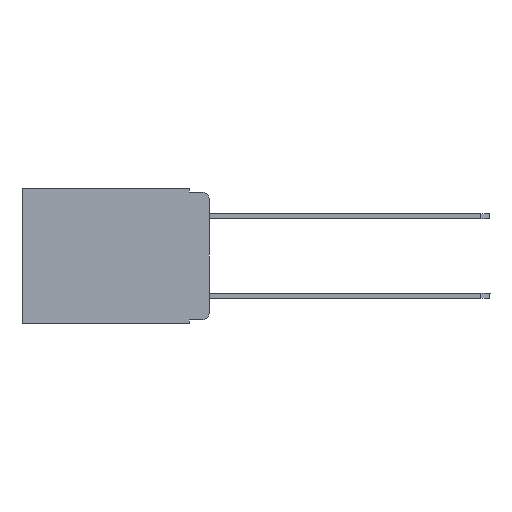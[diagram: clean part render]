
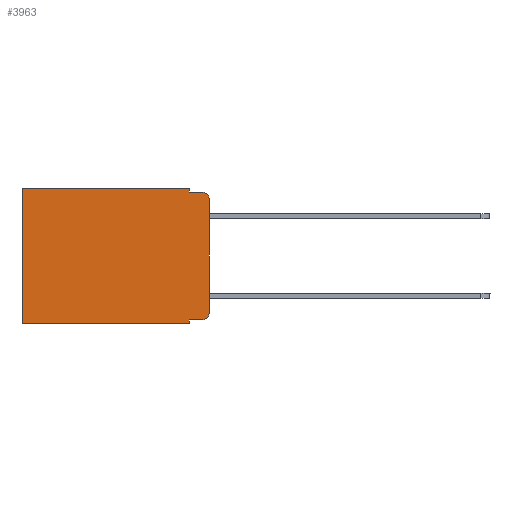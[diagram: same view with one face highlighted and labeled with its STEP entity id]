
A CAD part, left-side view. The second image highlights one B-rep face of the part: STEP entity #3963.
In plain terms, the highlighted planar face has unit normal (-1, 0, 0).
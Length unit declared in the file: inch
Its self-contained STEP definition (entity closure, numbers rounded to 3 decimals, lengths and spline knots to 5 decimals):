
#516 = DIRECTION ( 'NONE',  ( 0., -1., 0. ) ) ;
#684 = EDGE_CURVE ( 'NONE', #8232, #2446, #5012, .T. ) ;
#931 = DIRECTION ( 'NONE',  ( 0., 0., -1. ) ) ;
#959 = FACE_OUTER_BOUND ( 'NONE', #6966, .T. ) ;
#1146 = VERTEX_POINT ( 'NONE', #11413 ) ;
#1171 = AXIS2_PLACEMENT_3D ( 'NONE', #11766, #9076, #5073 ) ;
#1216 = ORIENTED_EDGE ( 'NONE', *, *, #16501, .T. ) ;
#1362 = EDGE_CURVE ( 'NONE', #7053, #8490, #6980, .T. ) ;
#1566 = ORIENTED_EDGE ( 'NONE', *, *, #14973, .T. ) ;
#1646 = VERTEX_POINT ( 'NONE', #10057 ) ;
#2324 = CARTESIAN_POINT ( 'NONE',  ( 0.298, 0.051, -0.01 ) ) ;
#2446 = VERTEX_POINT ( 'NONE', #9482 ) ;
#2644 = ORIENTED_EDGE ( 'NONE', *, *, #13585, .F. ) ;
#2721 = CARTESIAN_POINT ( 'NONE',  ( 0.298, 0., -0.313 ) ) ;
#3085 = CARTESIAN_POINT ( 'NONE',  ( 0.298, 0.051, 0. ) ) ;
#3963 = ADVANCED_FACE ( 'NONE', ( #959 ), #5052, .F. ) ;
#4472 = ORIENTED_EDGE ( 'NONE', *, *, #6833, .F. ) ;
#4945 = ORIENTED_EDGE ( 'NONE', *, *, #684, .T. ) ;
#5012 = LINE ( 'NONE', #15584, #7957 ) ;
#5049 = CARTESIAN_POINT ( 'NONE',  ( 0.298, 0., 0. ) ) ;
#5052 = PLANE ( 'NONE',  #6830 ) ;
#5073 = DIRECTION ( 'NONE',  ( 0., 0., -1. ) ) ;
#5092 = VECTOR ( 'NONE', #10422, 39.37008 ) ;
#5116 = CARTESIAN_POINT ( 'NONE',  ( 0.298, 0., 0. ) ) ;
#5578 = ORIENTED_EDGE ( 'NONE', *, *, #1362, .T. ) ;
#6239 = DIRECTION ( 'NONE',  ( 1., 0., 0. ) ) ;
#6269 = VECTOR ( 'NONE', #12137, 39.37008 ) ;
#6398 = DIRECTION ( 'NONE',  ( 0., -1., 0. ) ) ;
#6575 = CIRCLE ( 'NONE', #9666, 0.02 ) ;
#6630 = CARTESIAN_POINT ( 'NONE',  ( 0.298, 0., -0.03 ) ) ;
#6830 = AXIS2_PLACEMENT_3D ( 'NONE', #13055, #6239, #8967 ) ;
#6833 = EDGE_CURVE ( 'NONE', #8693, #1146, #7066, .T. ) ;
#6857 = EDGE_CURVE ( 'NONE', #13634, #15455, #14972, .T. ) ;
#6965 = VECTOR ( 'NONE', #516, 39.37008 ) ;
#6966 = EDGE_LOOP ( 'NONE', ( #12367, #15960, #10070, #8259, #1216, #4945, #2644, #4472, #1566, #5578 ) ) ;
#6980 = CIRCLE ( 'NONE', #1171, 0.02 ) ;
#7053 = VERTEX_POINT ( 'NONE', #15808 ) ;
#7066 = LINE ( 'NONE', #3085, #6269 ) ;
#7824 = DIRECTION ( 'NONE',  ( 0., 0., -1. ) ) ;
#7957 = VECTOR ( 'NONE', #11342, 39.37008 ) ;
#8232 = VERTEX_POINT ( 'NONE', #12311 ) ;
#8259 = ORIENTED_EDGE ( 'NONE', *, *, #6857, .F. ) ;
#8490 = VERTEX_POINT ( 'NONE', #2721 ) ;
#8693 = VERTEX_POINT ( 'NONE', #13674 ) ;
#8926 = VECTOR ( 'NONE', #7824, 39.37008 ) ;
#8967 = DIRECTION ( 'NONE',  ( 0., 0., -1. ) ) ;
#9021 = CARTESIAN_POINT ( 'NONE',  ( 0.298, 0.02, -0.03 ) ) ;
#9076 = DIRECTION ( 'NONE',  ( -1., 0., 0. ) ) ;
#9301 = EDGE_CURVE ( 'NONE', #17074, #1646, #6575, .T. ) ;
#9450 = VECTOR ( 'NONE', #11534, 39.37008 ) ;
#9482 = CARTESIAN_POINT ( 'NONE',  ( 0.298, 0.473, -0.343 ) ) ;
#9666 = AXIS2_PLACEMENT_3D ( 'NONE', #9021, #16882, #931 ) ;
#9917 = VECTOR ( 'NONE', #13995, 39.37008 ) ;
#10057 = CARTESIAN_POINT ( 'NONE',  ( 0.298, 0.02, -0.01 ) ) ;
#10070 = ORIENTED_EDGE ( 'NONE', *, *, #16459, .F. ) ;
#10422 = DIRECTION ( 'NONE',  ( 0., 1., 0. ) ) ;
#10907 = VECTOR ( 'NONE', #6398, 39.37008 ) ;
#11342 = DIRECTION ( 'NONE',  ( 0., 0., -1. ) ) ;
#11413 = CARTESIAN_POINT ( 'NONE',  ( 0.298, 0.051, -0.343 ) ) ;
#11452 = CARTESIAN_POINT ( 'NONE',  ( 0.298, 0., -0.343 ) ) ;
#11534 = DIRECTION ( 'NONE',  ( 0., 1., 0. ) ) ;
#11766 = CARTESIAN_POINT ( 'NONE',  ( 0.298, 0.02, -0.313 ) ) ;
#12137 = DIRECTION ( 'NONE',  ( 0., 0., -1. ) ) ;
#12311 = CARTESIAN_POINT ( 'NONE',  ( 0.298, 0.473, 0. ) ) ;
#12367 = ORIENTED_EDGE ( 'NONE', *, *, #14623, .F. ) ;
#12762 = LINE ( 'NONE', #11452, #9450 ) ;
#13055 = CARTESIAN_POINT ( 'NONE',  ( 0.298, 0., 0. ) ) ;
#13118 = LINE ( 'NONE', #2324, #10907 ) ;
#13585 = EDGE_CURVE ( 'NONE', #1146, #2446, #12762, .T. ) ;
#13634 = VERTEX_POINT ( 'NONE', #14231 ) ;
#13642 = CARTESIAN_POINT ( 'NONE',  ( 0.298, 0.051, -0.333 ) ) ;
#13674 = CARTESIAN_POINT ( 'NONE',  ( 0.298, 0.051, -0.333 ) ) ;
#13995 = DIRECTION ( 'NONE',  ( 0., 0., -1. ) ) ;
#14080 = LINE ( 'NONE', #5049, #8926 ) ;
#14231 = CARTESIAN_POINT ( 'NONE',  ( 0.298, 0.051, 0. ) ) ;
#14623 = EDGE_CURVE ( 'NONE', #17074, #8490, #14080, .T. ) ;
#14972 = LINE ( 'NONE', #16099, #9917 ) ;
#14973 = EDGE_CURVE ( 'NONE', #8693, #7053, #16392, .T. ) ;
#15235 = CARTESIAN_POINT ( 'NONE',  ( 0.298, 0.051, -0.01 ) ) ;
#15455 = VERTEX_POINT ( 'NONE', #15235 ) ;
#15584 = CARTESIAN_POINT ( 'NONE',  ( 0.298, 0.473, 0. ) ) ;
#15808 = CARTESIAN_POINT ( 'NONE',  ( 0.298, 0.02, -0.333 ) ) ;
#15960 = ORIENTED_EDGE ( 'NONE', *, *, #9301, .T. ) ;
#16099 = CARTESIAN_POINT ( 'NONE',  ( 0.298, 0.051, 0. ) ) ;
#16392 = LINE ( 'NONE', #13642, #6965 ) ;
#16459 = EDGE_CURVE ( 'NONE', #15455, #1646, #13118, .T. ) ;
#16501 = EDGE_CURVE ( 'NONE', #13634, #8232, #16978, .T. ) ;
#16882 = DIRECTION ( 'NONE',  ( -1., 0., 0. ) ) ;
#16978 = LINE ( 'NONE', #5116, #5092 ) ;
#17074 = VERTEX_POINT ( 'NONE', #6630 ) ;
